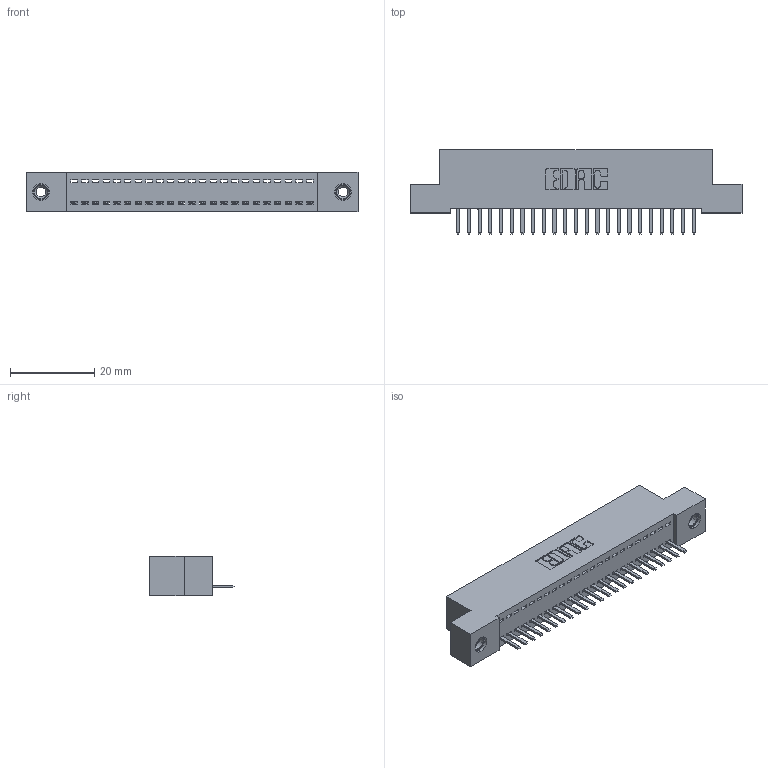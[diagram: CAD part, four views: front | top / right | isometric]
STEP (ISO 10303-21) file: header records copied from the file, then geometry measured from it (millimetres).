
FILE_DESCRIPTION (( 'STEP AP203' ), '1' );
FILE_NAME ('392-023-520-108.STEP', '2018-08-15T13:18:24', ( '' ), ( '' ), 'SwSTEP 2.0', 'SolidWorks 2016', '' );
FILE_SCHEMA (( 'CONFIG_CONTROL_DESIGN' ));
Length unit declared in the file: inch
Products named in the file (4): 342 Part_TI; 345-292-001_345-293-120; 345-250-001_345-250-003-102; 392-023-520-108
Assembly tree (26 placements, depth 2):
  392-023-520-108
    342 Part_TI
    345-292-001_345-293-120  x23
    345-250-001_345-250-003-102  x2
Bounding box: 78.74 x 20.02 x 9.4 mm (x, y, z)
Volume: 6762.1 mm3; surface area: 9381.3 mm2
Topology: 26 solids, 26 shells, 1596 faces, 4667 edges, 3042 vertices
Faces by surface type: plane 1110, cylinder 470, cone 12, torus 4
Entity records: 17686 total; most frequent: CARTESIAN_POINT 3046, ORIENTED_EDGE 2986, DIRECTION 2629, EDGE_CURVE 1493, VECTOR 1341, LINE 1341, VERTEX_POINT 988, AXIS2_PLACEMENT_3D 644
